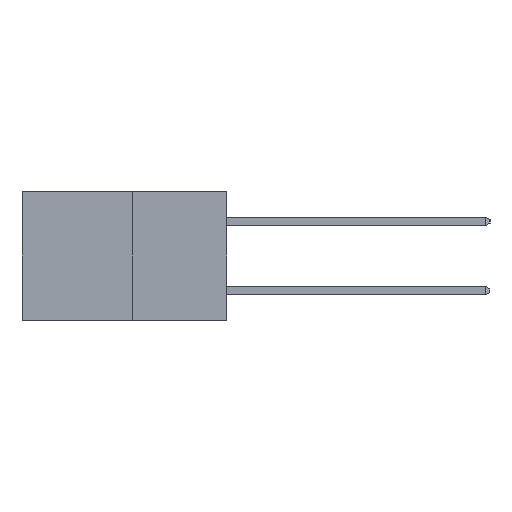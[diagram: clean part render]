
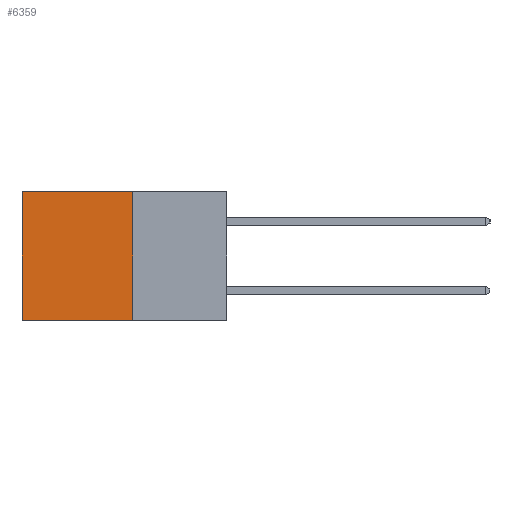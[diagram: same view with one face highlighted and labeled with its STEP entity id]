
A CAD part, left-side view. The second image highlights one B-rep face of the part: STEP entity #6359.
In plain terms, the highlighted planar face has unit normal (-1, 0, 0).
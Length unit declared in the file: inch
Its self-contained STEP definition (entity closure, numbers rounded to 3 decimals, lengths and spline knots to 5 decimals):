
#222 = DIRECTION ( 'NONE',  ( 0., 0., -1. ) ) ;
#573 = ORIENTED_EDGE ( 'NONE', *, *, #4408, .T. ) ;
#659 = DIRECTION ( 'NONE',  ( 0., 1., 0. ) ) ;
#1201 = FACE_OUTER_BOUND ( 'NONE', #17091, .T. ) ;
#1243 = VERTEX_POINT ( 'NONE', #4855 ) ;
#1252 = EDGE_CURVE ( 'NONE', #1243, #13583, #13246, .T. ) ;
#1743 = ORIENTED_EDGE ( 'NONE', *, *, #1252, .T. ) ;
#2049 = CARTESIAN_POINT ( 'NONE',  ( 0.277, 0.27, -0.37 ) ) ;
#2119 = VECTOR ( 'NONE', #3639, 39.37008 ) ;
#2462 = ORIENTED_EDGE ( 'NONE', *, *, #7180, .F. ) ;
#2464 = VECTOR ( 'NONE', #659, 39.37008 ) ;
#3265 = CARTESIAN_POINT ( 'NONE',  ( 0.277, 0.27, 0. ) ) ;
#3372 = VECTOR ( 'NONE', #4851, 39.37008 ) ;
#3639 = DIRECTION ( 'NONE',  ( 0., 1., 0. ) ) ;
#4408 = EDGE_CURVE ( 'NONE', #11346, #1243, #5763, .T. ) ;
#4851 = DIRECTION ( 'NONE',  ( 0., 0., -1. ) ) ;
#4855 = CARTESIAN_POINT ( 'NONE',  ( 0.277, 0.59, 0. ) ) ;
#5763 = LINE ( 'NONE', #3265, #2119 ) ;
#5867 = VECTOR ( 'NONE', #222, 39.37008 ) ;
#6359 = ADVANCED_FACE ( 'NONE', ( #1201 ), #11379, .F. ) ;
#7180 = EDGE_CURVE ( 'NONE', #11253, #13583, #9813, .T. ) ;
#7256 = DIRECTION ( 'NONE',  ( 1., 0., 0. ) ) ;
#9813 = LINE ( 'NONE', #13068, #2464 ) ;
#11253 = VERTEX_POINT ( 'NONE', #13323 ) ;
#11289 = CARTESIAN_POINT ( 'NONE',  ( 0.277, 0.59, -0.37 ) ) ;
#11346 = VERTEX_POINT ( 'NONE', #17563 ) ;
#11379 = PLANE ( 'NONE',  #11751 ) ;
#11751 = AXIS2_PLACEMENT_3D ( 'NONE', #15546, #7256, #16888 ) ;
#13068 = CARTESIAN_POINT ( 'NONE',  ( 0.277, 0.27, -0.37 ) ) ;
#13246 = LINE ( 'NONE', #14400, #5867 ) ;
#13323 = CARTESIAN_POINT ( 'NONE',  ( 0.277, 0.27, -0.37 ) ) ;
#13583 = VERTEX_POINT ( 'NONE', #11289 ) ;
#14400 = CARTESIAN_POINT ( 'NONE',  ( 0.277, 0.59, -0.37 ) ) ;
#15546 = CARTESIAN_POINT ( 'NONE',  ( 0.277, 0.27, -0.37 ) ) ;
#16135 = EDGE_CURVE ( 'NONE', #11346, #11253, #17120, .T. ) ;
#16888 = DIRECTION ( 'NONE',  ( 0., 0., -1. ) ) ;
#17091 = EDGE_LOOP ( 'NONE', ( #1743, #2462, #17111, #573 ) ) ;
#17111 = ORIENTED_EDGE ( 'NONE', *, *, #16135, .F. ) ;
#17120 = LINE ( 'NONE', #2049, #3372 ) ;
#17563 = CARTESIAN_POINT ( 'NONE',  ( 0.277, 0.27, 0. ) ) ;
